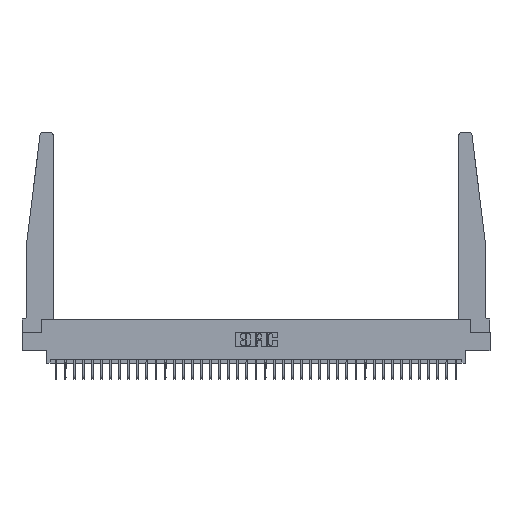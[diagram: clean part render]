
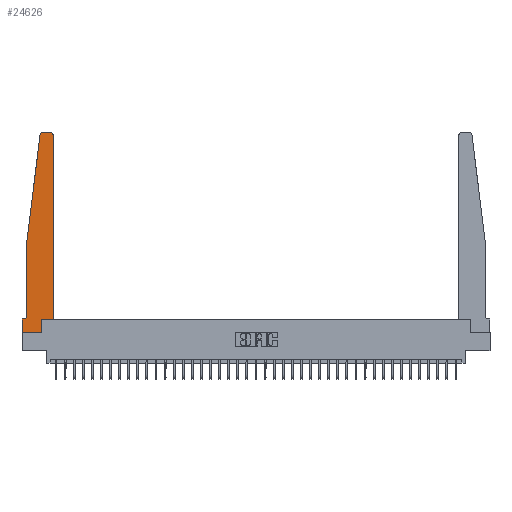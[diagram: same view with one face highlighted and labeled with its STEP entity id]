
A CAD part, top view. The second image highlights one B-rep face of the part: STEP entity #24626.
In plain terms, the highlighted planar face has unit normal (0, 0, 1).
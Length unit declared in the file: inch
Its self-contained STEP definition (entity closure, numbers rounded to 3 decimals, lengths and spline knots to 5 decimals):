
#124 = LINE ( 'NONE', #18833, #7129 ) ;
#295 = CIRCLE ( 'NONE', #11422, 0.05 ) ;
#661 = CARTESIAN_POINT ( 'NONE',  ( 0.395, 2.75, 0.37 ) ) ;
#996 = DIRECTION ( 'NONE',  ( 0., -1., 0. ) ) ;
#1592 = ORIENTED_EDGE ( 'NONE', *, *, #3207, .T. ) ;
#1597 = VECTOR ( 'NONE', #13006, 39.37008 ) ;
#1607 = CARTESIAN_POINT ( 'NONE',  ( 0.2605, 0.18, 0.37 ) ) ;
#1942 = DIRECTION ( 'NONE',  ( 0., 0., 1. ) ) ;
#2155 = VERTEX_POINT ( 'NONE', #26748 ) ;
#3052 = EDGE_CURVE ( 'NONE', #19724, #11979, #29033, .T. ) ;
#3207 = EDGE_CURVE ( 'NONE', #20062, #19724, #6205, .T. ) ;
#3604 = DIRECTION ( 'NONE',  ( -1., 0., 0. ) ) ;
#4012 = CARTESIAN_POINT ( 'NONE',  ( 0.065, 1.25, 0.37 ) ) ;
#4196 = DIRECTION ( 'NONE',  ( 1., 0., 0. ) ) ;
#4314 = VERTEX_POINT ( 'NONE', #26311 ) ;
#4944 = AXIS2_PLACEMENT_3D ( 'NONE', #21072, #32203, #26922 ) ;
#4963 = ORIENTED_EDGE ( 'NONE', *, *, #19581, .T. ) ;
#4965 = EDGE_CURVE ( 'NONE', #33111, #30205, #21678, .T. ) ;
#5073 = DIRECTION ( 'NONE',  ( 1., 0., 0. ) ) ;
#5483 = ORIENTED_EDGE ( 'NONE', *, *, #4965, .T. ) ;
#5690 = CARTESIAN_POINT ( 'NONE',  ( 0.065, 0.1875, 0.37 ) ) ;
#6205 = CIRCLE ( 'NONE', #24909, 0.03 ) ;
#6666 = CIRCLE ( 'NONE', #23005, 0.03 ) ;
#7083 = VERTEX_POINT ( 'NONE', #1607 ) ;
#7129 = VECTOR ( 'NONE', #35960, 39.37008 ) ;
#8567 = ORIENTED_EDGE ( 'NONE', *, *, #32435, .T. ) ;
#8793 = CARTESIAN_POINT ( 'NONE',  ( 0.015, 0.1875, 0.37 ) ) ;
#9232 = EDGE_LOOP ( 'NONE', ( #19252, #18314, #29242, #26378, #36006, #34547, #26194, #5483, #17371, #4963, #8567, #1592 ) ) ;
#10057 = DIRECTION ( 'NONE',  ( 0., -1., 0. ) ) ;
#10161 = VECTOR ( 'NONE', #10278, 39.37008 ) ;
#10172 = EDGE_CURVE ( 'NONE', #4314, #17418, #17931, .T. ) ;
#10278 = DIRECTION ( 'NONE',  ( -0.122, -0.992, 0. ) ) ;
#11126 = CARTESIAN_POINT ( 'NONE',  ( 0., 0., 0.37 ) ) ;
#11422 = AXIS2_PLACEMENT_3D ( 'NONE', #17580, #31629, #14998 ) ;
#11979 = VERTEX_POINT ( 'NONE', #35593 ) ;
#12051 = CARTESIAN_POINT ( 'NONE',  ( 0.25, 2.75, 0.37 ) ) ;
#13006 = DIRECTION ( 'NONE',  ( 0., 1., 0. ) ) ;
#13033 = LINE ( 'NONE', #24004, #10161 ) ;
#13371 = LINE ( 'NONE', #15743, #1597 ) ;
#13566 = DIRECTION ( 'NONE',  ( -1., 0., 0. ) ) ;
#13806 = VERTEX_POINT ( 'NONE', #16762 ) ;
#14104 = DIRECTION ( 'NONE',  ( 0., 1., 0. ) ) ;
#14998 = DIRECTION ( 'NONE',  ( -1., 0., 0. ) ) ;
#15743 = CARTESIAN_POINT ( 'NONE',  ( 0.425, 0.18, 0.37 ) ) ;
#15832 = DIRECTION ( 'NONE',  ( 1., 0., 0. ) ) ;
#16307 = PLANE ( 'NONE',  #4944 ) ;
#16483 = VECTOR ( 'NONE', #13566, 39.37008 ) ;
#16762 = CARTESIAN_POINT ( 'NONE',  ( 0.24675, 2.72367, 0.37 ) ) ;
#17371 = ORIENTED_EDGE ( 'NONE', *, *, #25808, .T. ) ;
#17418 = VERTEX_POINT ( 'NONE', #18935 ) ;
#17580 = CARTESIAN_POINT ( 'NONE',  ( 0.015, 0.2375, 0.37 ) ) ;
#17931 = LINE ( 'NONE', #4012, #33600 ) ;
#18118 = DIRECTION ( 'NONE',  ( 0., 0., 1. ) ) ;
#18314 = ORIENTED_EDGE ( 'NONE', *, *, #25920, .T. ) ;
#18833 = CARTESIAN_POINT ( 'NONE',  ( 0.425, 0.18, 0.37 ) ) ;
#18935 = CARTESIAN_POINT ( 'NONE',  ( 0.065, 0.2375, 0.37 ) ) ;
#19151 = EDGE_CURVE ( 'NONE', #20559, #2155, #36003, .T. ) ;
#19160 = VECTOR ( 'NONE', #996, 39.37008 ) ;
#19252 = ORIENTED_EDGE ( 'NONE', *, *, #3052, .T. ) ;
#19581 = EDGE_CURVE ( 'NONE', #7083, #31619, #124, .T. ) ;
#19724 = VERTEX_POINT ( 'NONE', #661 ) ;
#20062 = VERTEX_POINT ( 'NONE', #33491 ) ;
#20559 = VERTEX_POINT ( 'NONE', #8793 ) ;
#21072 = CARTESIAN_POINT ( 'NONE',  ( 0., 0.1875, 0.37 ) ) ;
#21496 = CARTESIAN_POINT ( 'NONE',  ( 0., 0., 0.37 ) ) ;
#21678 = LINE ( 'NONE', #21496, #34052 ) ;
#21797 = EDGE_CURVE ( 'NONE', #17418, #20559, #295, .T. ) ;
#22794 = CARTESIAN_POINT ( 'NONE',  ( 0., 0., 0.37 ) ) ;
#23005 = AXIS2_PLACEMENT_3D ( 'NONE', #31978, #18118, #4196 ) ;
#23013 = CARTESIAN_POINT ( 'NONE',  ( 0.425, 0.18, 0.37 ) ) ;
#24004 = CARTESIAN_POINT ( 'NONE',  ( 0.065, 1.25, 0.37 ) ) ;
#24177 = VECTOR ( 'NONE', #14104, 39.37008 ) ;
#24626 = ADVANCED_FACE ( 'NONE', ( #30185 ), #16307, .T. ) ;
#24909 = AXIS2_PLACEMENT_3D ( 'NONE', #26649, #1942, #5073 ) ;
#25646 = EDGE_CURVE ( 'NONE', #13806, #4314, #13033, .T. ) ;
#25808 = EDGE_CURVE ( 'NONE', #30205, #7083, #27997, .T. ) ;
#25920 = EDGE_CURVE ( 'NONE', #11979, #13806, #6666, .T. ) ;
#26194 = ORIENTED_EDGE ( 'NONE', *, *, #32039, .T. ) ;
#26311 = CARTESIAN_POINT ( 'NONE',  ( 0.065, 1.25, 0.37 ) ) ;
#26378 = ORIENTED_EDGE ( 'NONE', *, *, #10172, .T. ) ;
#26649 = CARTESIAN_POINT ( 'NONE',  ( 0.395, 2.72, 0.37 ) ) ;
#26696 = VECTOR ( 'NONE', #3604, 39.37008 ) ;
#26748 = CARTESIAN_POINT ( 'NONE',  ( 0., 0.1875, 0.37 ) ) ;
#26922 = DIRECTION ( 'NONE',  ( 1., 0., 0. ) ) ;
#27814 = CARTESIAN_POINT ( 'NONE',  ( 0.2605, 0.18, 0.37 ) ) ;
#27997 = LINE ( 'NONE', #27814, #24177 ) ;
#29033 = LINE ( 'NONE', #12051, #26696 ) ;
#29242 = ORIENTED_EDGE ( 'NONE', *, *, #25646, .T. ) ;
#30185 = FACE_OUTER_BOUND ( 'NONE', #9232, .T. ) ;
#30205 = VERTEX_POINT ( 'NONE', #30408 ) ;
#30408 = CARTESIAN_POINT ( 'NONE',  ( 0.2605, 0., 0.37 ) ) ;
#31619 = VERTEX_POINT ( 'NONE', #23013 ) ;
#31629 = DIRECTION ( 'NONE',  ( 0., 0., -1. ) ) ;
#31713 = LINE ( 'NONE', #22794, #19160 ) ;
#31978 = CARTESIAN_POINT ( 'NONE',  ( 0.27653, 2.72, 0.37 ) ) ;
#32039 = EDGE_CURVE ( 'NONE', #2155, #33111, #31713, .T. ) ;
#32203 = DIRECTION ( 'NONE',  ( 0., 0., 1. ) ) ;
#32435 = EDGE_CURVE ( 'NONE', #31619, #20062, #13371, .T. ) ;
#33111 = VERTEX_POINT ( 'NONE', #11126 ) ;
#33491 = CARTESIAN_POINT ( 'NONE',  ( 0.425, 2.72, 0.37 ) ) ;
#33600 = VECTOR ( 'NONE', #10057, 39.37008 ) ;
#34052 = VECTOR ( 'NONE', #15832, 39.37008 ) ;
#34547 = ORIENTED_EDGE ( 'NONE', *, *, #19151, .T. ) ;
#35593 = CARTESIAN_POINT ( 'NONE',  ( 0.27653, 2.75, 0.37 ) ) ;
#35960 = DIRECTION ( 'NONE',  ( 1., 0., 0. ) ) ;
#36003 = LINE ( 'NONE', #5690, #16483 ) ;
#36006 = ORIENTED_EDGE ( 'NONE', *, *, #21797, .T. ) ;
